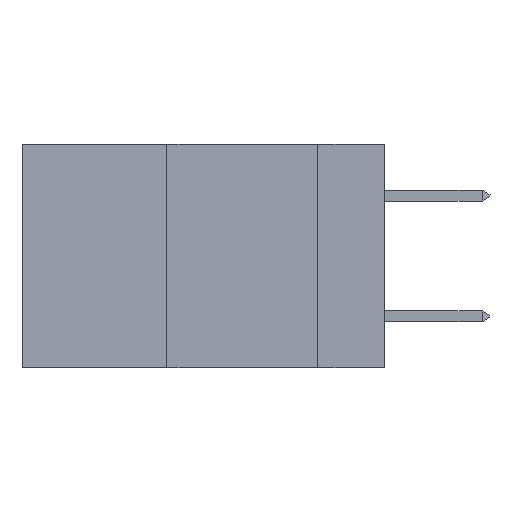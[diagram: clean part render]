
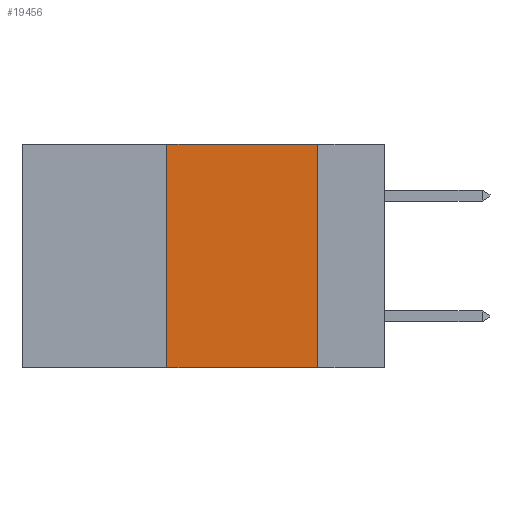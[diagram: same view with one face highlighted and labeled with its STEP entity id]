
A CAD part, left-side view. The second image highlights one B-rep face of the part: STEP entity #19456.
In plain terms, the highlighted planar face has unit normal (-1, 0, 0).
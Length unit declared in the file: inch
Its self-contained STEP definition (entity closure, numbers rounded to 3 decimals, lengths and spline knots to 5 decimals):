
#496 = EDGE_LOOP ( 'NONE', ( #8508, #4238, #5672, #6230 ) ) ;
#1332 = EDGE_CURVE ( 'NONE', #11824, #17546, #14447, .T. ) ;
#1776 = VERTEX_POINT ( 'NONE', #22356 ) ;
#2604 = CARTESIAN_POINT ( 'NONE',  ( 0., 0.11, -0.37 ) ) ;
#3238 = VECTOR ( 'NONE', #5244, 39.37008 ) ;
#4238 = ORIENTED_EDGE ( 'NONE', *, *, #18567, .F. ) ;
#5244 = DIRECTION ( 'NONE',  ( 0., -1., 0. ) ) ;
#5672 = ORIENTED_EDGE ( 'NONE', *, *, #12374, .F. ) ;
#6230 = ORIENTED_EDGE ( 'NONE', *, *, #1332, .T. ) ;
#6327 = DIRECTION ( 'NONE',  ( 0., 0., -1. ) ) ;
#7048 = CARTESIAN_POINT ( 'NONE',  ( 0., 0.11, 0. ) ) ;
#8508 = ORIENTED_EDGE ( 'NONE', *, *, #18798, .F. ) ;
#9541 = DIRECTION ( 'NONE',  ( 0., -1., 0. ) ) ;
#10277 = DIRECTION ( 'NONE',  ( 1., 0., 0. ) ) ;
#11824 = VERTEX_POINT ( 'NONE', #21281 ) ;
#12374 = EDGE_CURVE ( 'NONE', #11824, #1776, #18120, .T. ) ;
#13012 = VERTEX_POINT ( 'NONE', #7048 ) ;
#13149 = CARTESIAN_POINT ( 'NONE',  ( 0., 0.36, 0. ) ) ;
#14026 = LINE ( 'NONE', #18316, #24741 ) ;
#14179 = PLANE ( 'NONE',  #18656 ) ;
#14447 = LINE ( 'NONE', #15224, #3238 ) ;
#15224 = CARTESIAN_POINT ( 'NONE',  ( 0., 0.6, -0.37 ) ) ;
#15598 = LINE ( 'NONE', #17509, #19769 ) ;
#17458 = VECTOR ( 'NONE', #25193, 39.37008 ) ;
#17509 = CARTESIAN_POINT ( 'NONE',  ( 0., 0.6, 0. ) ) ;
#17546 = VERTEX_POINT ( 'NONE', #2604 ) ;
#18120 = LINE ( 'NONE', #13149, #17458 ) ;
#18316 = CARTESIAN_POINT ( 'NONE',  ( 0., 0.11, 0. ) ) ;
#18567 = EDGE_CURVE ( 'NONE', #1776, #13012, #15598, .T. ) ;
#18656 = AXIS2_PLACEMENT_3D ( 'NONE', #22300, #10277, #24319 ) ;
#18798 = EDGE_CURVE ( 'NONE', #13012, #17546, #14026, .T. ) ;
#19456 = ADVANCED_FACE ( 'NONE', ( #24395 ), #14179, .F. ) ;
#19769 = VECTOR ( 'NONE', #9541, 39.37008 ) ;
#21281 = CARTESIAN_POINT ( 'NONE',  ( 0., 0.36, -0.37 ) ) ;
#22300 = CARTESIAN_POINT ( 'NONE',  ( 0., 0.6, 0. ) ) ;
#22356 = CARTESIAN_POINT ( 'NONE',  ( 0., 0.36, 0. ) ) ;
#24319 = DIRECTION ( 'NONE',  ( 0., 0., -1. ) ) ;
#24395 = FACE_OUTER_BOUND ( 'NONE', #496, .T. ) ;
#24741 = VECTOR ( 'NONE', #6327, 39.37008 ) ;
#25193 = DIRECTION ( 'NONE',  ( 0., 0., 1. ) ) ;
